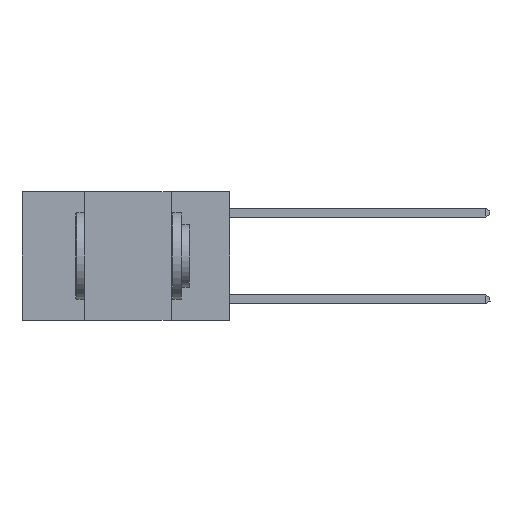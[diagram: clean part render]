
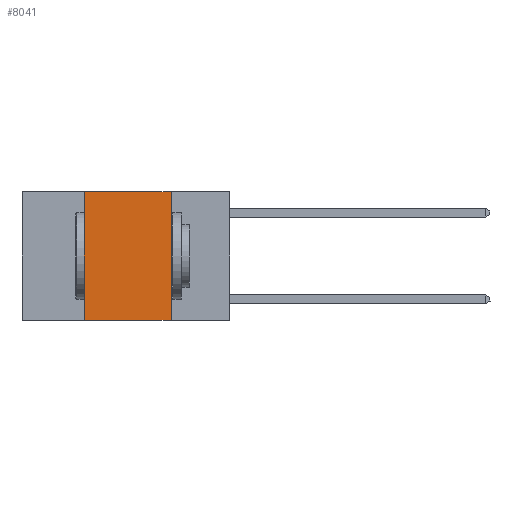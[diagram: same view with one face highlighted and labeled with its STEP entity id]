
A CAD part, left-side view. The second image highlights one B-rep face of the part: STEP entity #8041.
In plain terms, the highlighted planar face has unit normal (-1, 0, 0).
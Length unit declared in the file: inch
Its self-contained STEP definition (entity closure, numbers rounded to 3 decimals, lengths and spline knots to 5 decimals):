
#79 = DIRECTION ( 'NONE',  ( 0., 0., -1. ) ) ;
#978 = VERTEX_POINT ( 'NONE', #1686 ) ;
#1015 = DIRECTION ( 'NONE',  ( 0., 0., -1. ) ) ;
#1132 = VECTOR ( 'NONE', #1260, 39.37008 ) ;
#1260 = DIRECTION ( 'NONE',  ( 0., -1., 0. ) ) ;
#1626 = EDGE_CURVE ( 'NONE', #3607, #978, #2640, .T. ) ;
#1686 = CARTESIAN_POINT ( 'NONE',  ( 0., 0.17, -0.37 ) ) ;
#1891 = DIRECTION ( 'NONE',  ( 0., 0., 1. ) ) ;
#2640 = LINE ( 'NONE', #3375, #6722 ) ;
#2729 = CARTESIAN_POINT ( 'NONE',  ( 0., 0.42, 0. ) ) ;
#3375 = CARTESIAN_POINT ( 'NONE',  ( 0., 0.17, 0. ) ) ;
#3409 = CARTESIAN_POINT ( 'NONE',  ( 0., 0.42, 0. ) ) ;
#3607 = VERTEX_POINT ( 'NONE', #7285 ) ;
#3838 = FACE_OUTER_BOUND ( 'NONE', #10219, .T. ) ;
#4193 = PLANE ( 'NONE',  #6982 ) ;
#4248 = VERTEX_POINT ( 'NONE', #3409 ) ;
#4323 = ORIENTED_EDGE ( 'NONE', *, *, #1626, .F. ) ;
#4325 = DIRECTION ( 'NONE',  ( 0., -1., 0. ) ) ;
#4333 = LINE ( 'NONE', #2729, #6239 ) ;
#4435 = ORIENTED_EDGE ( 'NONE', *, *, #8927, .T. ) ;
#4510 = ORIENTED_EDGE ( 'NONE', *, *, #9971, .F. ) ;
#4986 = DIRECTION ( 'NONE',  ( 1., 0., 0. ) ) ;
#5525 = VERTEX_POINT ( 'NONE', #7379 ) ;
#6155 = CARTESIAN_POINT ( 'NONE',  ( 0., 0.6, -0.37 ) ) ;
#6239 = VECTOR ( 'NONE', #1891, 39.37008 ) ;
#6254 = EDGE_CURVE ( 'NONE', #4248, #3607, #7531, .T. ) ;
#6722 = VECTOR ( 'NONE', #1015, 39.37008 ) ;
#6982 = AXIS2_PLACEMENT_3D ( 'NONE', #9781, #4986, #79 ) ;
#7197 = ORIENTED_EDGE ( 'NONE', *, *, #6254, .F. ) ;
#7285 = CARTESIAN_POINT ( 'NONE',  ( 0., 0.17, 0. ) ) ;
#7379 = CARTESIAN_POINT ( 'NONE',  ( 0., 0.42, -0.37 ) ) ;
#7531 = LINE ( 'NONE', #8359, #9531 ) ;
#8041 = ADVANCED_FACE ( 'NONE', ( #3838 ), #4193, .F. ) ;
#8359 = CARTESIAN_POINT ( 'NONE',  ( 0., 0.6, 0. ) ) ;
#8927 = EDGE_CURVE ( 'NONE', #5525, #978, #9484, .T. ) ;
#9484 = LINE ( 'NONE', #6155, #1132 ) ;
#9531 = VECTOR ( 'NONE', #4325, 39.37008 ) ;
#9781 = CARTESIAN_POINT ( 'NONE',  ( 0., 0.6, 0. ) ) ;
#9971 = EDGE_CURVE ( 'NONE', #5525, #4248, #4333, .T. ) ;
#10219 = EDGE_LOOP ( 'NONE', ( #4323, #7197, #4510, #4435 ) ) ;
